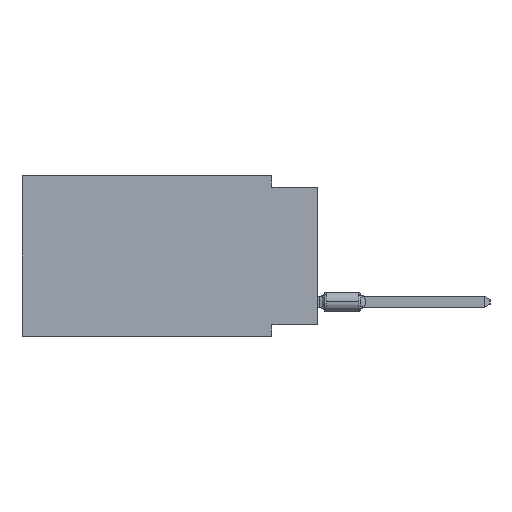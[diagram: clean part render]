
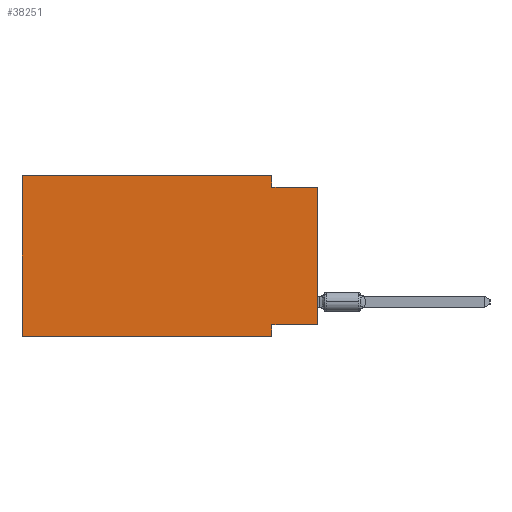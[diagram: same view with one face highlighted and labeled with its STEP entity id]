
A CAD part, left-side view. The second image highlights one B-rep face of the part: STEP entity #38251.
In plain terms, the highlighted planar face has unit normal (-1, 0, 0).
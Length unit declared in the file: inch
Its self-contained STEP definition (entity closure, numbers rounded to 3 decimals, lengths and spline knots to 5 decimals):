
#61 = ORIENTED_EDGE ( 'NONE', *, *, #46014, .F. ) ;
#1635 = EDGE_CURVE ( 'NONE', #64090, #60895, #62683, .T. ) ;
#2868 = VECTOR ( 'NONE', #50676, 39.37008 ) ;
#3747 = ORIENTED_EDGE ( 'NONE', *, *, #33011, .F. ) ;
#3851 = CARTESIAN_POINT ( 'NONE',  ( 0., 0., -0.025 ) ) ;
#4016 = ORIENTED_EDGE ( 'NONE', *, *, #19914, .F. ) ;
#5479 = CARTESIAN_POINT ( 'NONE',  ( 0., 0.1, -0.325 ) ) ;
#6365 = PLANE ( 'NONE',  #36747 ) ;
#6664 = ORIENTED_EDGE ( 'NONE', *, *, #22232, .F. ) ;
#7117 = DIRECTION ( 'NONE',  ( 0., 1., 0. ) ) ;
#7332 = DIRECTION ( 'NONE',  ( 0., 0., -1. ) ) ;
#8229 = CARTESIAN_POINT ( 'NONE',  ( 0., 0.1, -0.025 ) ) ;
#8745 = CARTESIAN_POINT ( 'NONE',  ( 0., 0., 0. ) ) ;
#10016 = DIRECTION ( 'NONE',  ( 0., -1., 0. ) ) ;
#11142 = DIRECTION ( 'NONE',  ( 0., 0., -1. ) ) ;
#11514 = CARTESIAN_POINT ( 'NONE',  ( 0., 0.1, 0. ) ) ;
#11553 = CARTESIAN_POINT ( 'NONE',  ( 0., 0., -0.325 ) ) ;
#12218 = CARTESIAN_POINT ( 'NONE',  ( 0., 0.645, 0. ) ) ;
#13213 = EDGE_CURVE ( 'NONE', #35564, #45084, #18256, .T. ) ;
#14175 = ORIENTED_EDGE ( 'NONE', *, *, #1635, .T. ) ;
#16478 = LINE ( 'NONE', #31867, #26160 ) ;
#16675 = CARTESIAN_POINT ( 'NONE',  ( 0., 0.645, 0. ) ) ;
#18256 = LINE ( 'NONE', #3851, #61606 ) ;
#18586 = VERTEX_POINT ( 'NONE', #5479 ) ;
#19914 = EDGE_CURVE ( 'NONE', #18586, #60895, #16478, .T. ) ;
#22232 = EDGE_CURVE ( 'NONE', #64090, #45526, #64734, .T. ) ;
#23229 = ORIENTED_EDGE ( 'NONE', *, *, #63355, .T. ) ;
#24659 = CARTESIAN_POINT ( 'NONE',  ( 0., 0.645, 0. ) ) ;
#25957 = DIRECTION ( 'NONE',  ( 0., -1., 0. ) ) ;
#26160 = VECTOR ( 'NONE', #11142, 39.37008 ) ;
#27350 = EDGE_LOOP ( 'NONE', ( #23229, #51902, #50761, #3747, #6664, #14175, #4016, #61 ) ) ;
#28746 = VECTOR ( 'NONE', #25957, 39.37008 ) ;
#31867 = CARTESIAN_POINT ( 'NONE',  ( 0., 0.1, -0.35 ) ) ;
#32359 = CARTESIAN_POINT ( 'NONE',  ( 0., 0.645, -0.35 ) ) ;
#33011 = EDGE_CURVE ( 'NONE', #45526, #57142, #54457, .T. ) ;
#35564 = VERTEX_POINT ( 'NONE', #8229 ) ;
#36747 = AXIS2_PLACEMENT_3D ( 'NONE', #16675, #58072, #7332 ) ;
#37090 = FACE_OUTER_BOUND ( 'NONE', #27350, .T. ) ;
#37895 = LINE ( 'NONE', #11514, #64850 ) ;
#38251 = ADVANCED_FACE ( 'NONE', ( #37090 ), #6365, .F. ) ;
#39948 = DIRECTION ( 'NONE',  ( 0., -1., 0. ) ) ;
#42894 = LINE ( 'NONE', #52565, #50215 ) ;
#45084 = VERTEX_POINT ( 'NONE', #51345 ) ;
#45526 = VERTEX_POINT ( 'NONE', #12218 ) ;
#46014 = EDGE_CURVE ( 'NONE', #61524, #18586, #42894, .T. ) ;
#49954 = VECTOR ( 'NONE', #10016, 39.37008 ) ;
#50215 = VECTOR ( 'NONE', #7117, 39.37008 ) ;
#50676 = DIRECTION ( 'NONE',  ( 0., 0., 1. ) ) ;
#50761 = ORIENTED_EDGE ( 'NONE', *, *, #56344, .F. ) ;
#51345 = CARTESIAN_POINT ( 'NONE',  ( 0., 0., -0.025 ) ) ;
#51902 = ORIENTED_EDGE ( 'NONE', *, *, #13213, .F. ) ;
#52565 = CARTESIAN_POINT ( 'NONE',  ( 0., 0., -0.325 ) ) ;
#54457 = LINE ( 'NONE', #64819, #49954 ) ;
#55147 = CARTESIAN_POINT ( 'NONE',  ( 0., 0.1, -0.35 ) ) ;
#55153 = DIRECTION ( 'NONE',  ( 0., 0., 1. ) ) ;
#56344 = EDGE_CURVE ( 'NONE', #57142, #35564, #37895, .T. ) ;
#57142 = VERTEX_POINT ( 'NONE', #64422 ) ;
#58072 = DIRECTION ( 'NONE',  ( 1., 0., 0. ) ) ;
#58228 = DIRECTION ( 'NONE',  ( 0., 0., -1. ) ) ;
#60895 = VERTEX_POINT ( 'NONE', #55147 ) ;
#61524 = VERTEX_POINT ( 'NONE', #11553 ) ;
#61606 = VECTOR ( 'NONE', #39948, 39.37008 ) ;
#62034 = CARTESIAN_POINT ( 'NONE',  ( 0., 0.645, -0.35 ) ) ;
#62683 = LINE ( 'NONE', #62034, #28746 ) ;
#63355 = EDGE_CURVE ( 'NONE', #61524, #45084, #65857, .T. ) ;
#64090 = VERTEX_POINT ( 'NONE', #32359 ) ;
#64310 = VECTOR ( 'NONE', #55153, 39.37008 ) ;
#64422 = CARTESIAN_POINT ( 'NONE',  ( 0., 0.1, 0. ) ) ;
#64734 = LINE ( 'NONE', #24659, #2868 ) ;
#64819 = CARTESIAN_POINT ( 'NONE',  ( 0., 0.645, 0. ) ) ;
#64850 = VECTOR ( 'NONE', #58228, 39.37008 ) ;
#65857 = LINE ( 'NONE', #8745, #64310 ) ;
